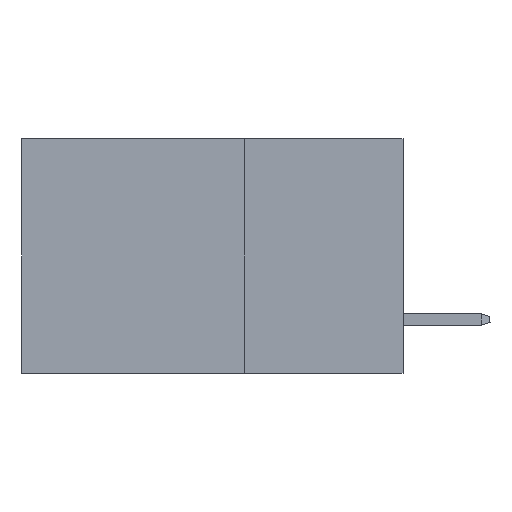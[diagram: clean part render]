
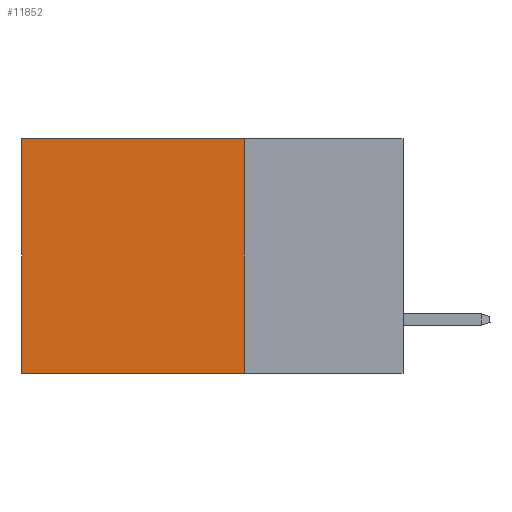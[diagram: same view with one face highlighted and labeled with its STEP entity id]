
A CAD part, left-side view. The second image highlights one B-rep face of the part: STEP entity #11852.
In plain terms, the highlighted planar face has unit normal (-1, 0, 0).
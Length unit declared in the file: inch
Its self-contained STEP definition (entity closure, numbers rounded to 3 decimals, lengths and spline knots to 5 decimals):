
#224 = VECTOR ( 'NONE', #15382, 39.37008 ) ;
#400 = VERTEX_POINT ( 'NONE', #16087 ) ;
#411 = VECTOR ( 'NONE', #10100, 39.37008 ) ;
#655 = LINE ( 'NONE', #18509, #7942 ) ;
#1179 = DIRECTION ( 'NONE',  ( 0., 0., -1. ) ) ;
#1914 = EDGE_LOOP ( 'NONE', ( #15145, #11036, #14845, #13928 ) ) ;
#2434 = EDGE_CURVE ( 'NONE', #11615, #400, #3413, .T. ) ;
#3413 = LINE ( 'NONE', #9408, #224 ) ;
#3979 = EDGE_CURVE ( 'NONE', #400, #13147, #15091, .T. ) ;
#4687 = DIRECTION ( 'NONE',  ( 0., 0., -1. ) ) ;
#4702 = CARTESIAN_POINT ( 'NONE',  ( 0.2875, 0.25, 0. ) ) ;
#5469 = PLANE ( 'NONE',  #11957 ) ;
#6441 = CARTESIAN_POINT ( 'NONE',  ( 0.2875, 0.6, 0. ) ) ;
#6683 = VERTEX_POINT ( 'NONE', #10065 ) ;
#7503 = CARTESIAN_POINT ( 'NONE',  ( 0.2875, 0.6, -0.37 ) ) ;
#7942 = VECTOR ( 'NONE', #9650, 39.37008 ) ;
#8512 = LINE ( 'NONE', #19047, #411 ) ;
#9408 = CARTESIAN_POINT ( 'NONE',  ( 0.2875, 0.25, 0. ) ) ;
#9650 = DIRECTION ( 'NONE',  ( 0., 1., 0. ) ) ;
#10065 = CARTESIAN_POINT ( 'NONE',  ( 0.2875, 0.25, -0.37 ) ) ;
#10100 = DIRECTION ( 'NONE',  ( 0., 0., -1. ) ) ;
#11036 = ORIENTED_EDGE ( 'NONE', *, *, #15709, .F. ) ;
#11615 = VERTEX_POINT ( 'NONE', #4702 ) ;
#11852 = ADVANCED_FACE ( 'NONE', ( #17416 ), #5469, .F. ) ;
#11868 = EDGE_CURVE ( 'NONE', #11615, #6683, #8512, .T. ) ;
#11957 = AXIS2_PLACEMENT_3D ( 'NONE', #13116, #16157, #1179 ) ;
#13116 = CARTESIAN_POINT ( 'NONE',  ( 0.2875, 0.25, 0. ) ) ;
#13147 = VERTEX_POINT ( 'NONE', #7503 ) ;
#13488 = VECTOR ( 'NONE', #4687, 39.37008 ) ;
#13928 = ORIENTED_EDGE ( 'NONE', *, *, #2434, .T. ) ;
#14845 = ORIENTED_EDGE ( 'NONE', *, *, #11868, .F. ) ;
#15091 = LINE ( 'NONE', #6441, #13488 ) ;
#15145 = ORIENTED_EDGE ( 'NONE', *, *, #3979, .T. ) ;
#15382 = DIRECTION ( 'NONE',  ( 0., 1., 0. ) ) ;
#15709 = EDGE_CURVE ( 'NONE', #6683, #13147, #655, .T. ) ;
#16087 = CARTESIAN_POINT ( 'NONE',  ( 0.2875, 0.6, 0. ) ) ;
#16157 = DIRECTION ( 'NONE',  ( 1., 0., 0. ) ) ;
#17416 = FACE_OUTER_BOUND ( 'NONE', #1914, .T. ) ;
#18509 = CARTESIAN_POINT ( 'NONE',  ( 0.2875, 0.25, -0.37 ) ) ;
#19047 = CARTESIAN_POINT ( 'NONE',  ( 0.2875, 0.25, 0. ) ) ;
